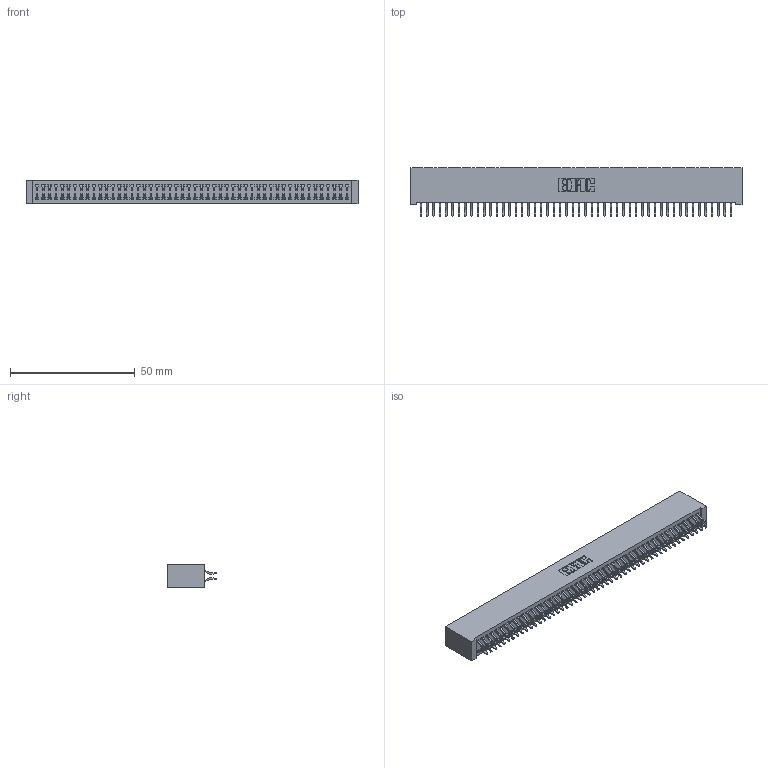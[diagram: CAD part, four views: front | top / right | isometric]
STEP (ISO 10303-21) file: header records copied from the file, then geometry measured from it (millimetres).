
FILE_DESCRIPTION (( 'STEP AP203' ), '1' );
FILE_NAME ('342-100-556-201.STEP', '2019-10-04T17:48:35', ( '' ), ( '' ), 'SwSTEP 2.0', 'SolidWorks 2016', '' );
FILE_SCHEMA (( 'CONFIG_CONTROL_DESIGN' ));
Length unit declared in the file: inch
Products named in the file (3): 342 Part_Lugless; 345-292-001_556 Tail; 342-100-556-201
Assembly tree (101 placements, depth 2):
  342-100-556-201
    342 Part_Lugless
    345-292-001_556 Tail  x100
Bounding box: 133.25 x 19.58 x 9.4 mm (x, y, z)
Volume: 12447.2 mm3; surface area: 20807.3 mm2
Topology: 101 solids, 101 shells, 5902 faces, 17575 edges, 11582 vertices
Faces by surface type: plane 4062, cylinder 1840
Entity records: 30943 total; most frequent: CARTESIAN_POINT 5130, ORIENTED_EDGE 5054, DIRECTION 4351, EDGE_CURVE 2527, LINE 2399, VECTOR 2399, VERTEX_POINT 1682, AXIS2_PLACEMENT_3D 976
